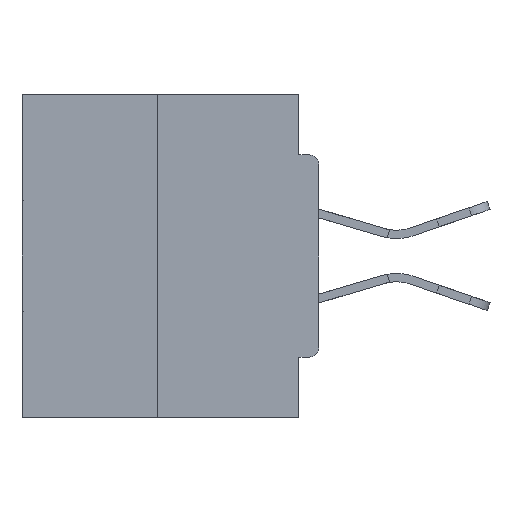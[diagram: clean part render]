
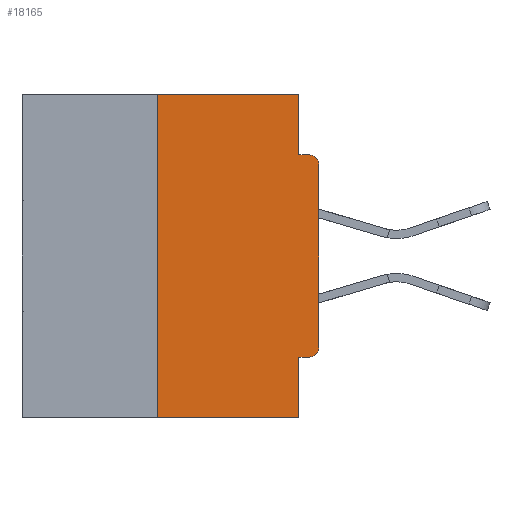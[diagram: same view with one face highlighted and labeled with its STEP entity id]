
A CAD part, left-side view. The second image highlights one B-rep face of the part: STEP entity #18165.
In plain terms, the highlighted planar face has unit normal (-1, 0, 0).
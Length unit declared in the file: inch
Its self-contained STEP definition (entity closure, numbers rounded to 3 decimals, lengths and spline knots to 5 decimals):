
#96 = VERTEX_POINT ( 'NONE', #27990 ) ;
#500 = DIRECTION ( 'NONE',  ( 0., -1., 0. ) ) ;
#645 = CIRCLE ( 'NONE', #2273, 0.015 ) ;
#762 = VECTOR ( 'NONE', #500, 39.37008 ) ;
#805 = VERTEX_POINT ( 'NONE', #32834 ) ;
#1297 = EDGE_CURVE ( 'NONE', #8215, #9489, #29503, .T. ) ;
#1760 = LINE ( 'NONE', #36639, #36650 ) ;
#1950 = EDGE_LOOP ( 'NONE', ( #38988, #21185, #4575, #33597, #34067, #13306, #17500, #25959, #10683, #33897 ) ) ;
#2273 = AXIS2_PLACEMENT_3D ( 'NONE', #25875, #7058, #6912 ) ;
#2349 = VERTEX_POINT ( 'NONE', #29491 ) ;
#2545 = VERTEX_POINT ( 'NONE', #11940 ) ;
#2670 = DIRECTION ( 'NONE',  ( 0., 0., -1. ) ) ;
#4311 = EDGE_CURVE ( 'NONE', #2545, #2349, #1760, .T. ) ;
#4575 = ORIENTED_EDGE ( 'NONE', *, *, #1297, .T. ) ;
#5375 = PLANE ( 'NONE',  #36277 ) ;
#5577 = AXIS2_PLACEMENT_3D ( 'NONE', #35127, #19532, #7070 ) ;
#5685 = LINE ( 'NONE', #37284, #11078 ) ;
#5915 = DIRECTION ( 'NONE',  ( 0., 0., 1. ) ) ;
#6201 = DIRECTION ( 'NONE',  ( 0., 1., 0. ) ) ;
#6490 = VECTOR ( 'NONE', #2670, 39.37008 ) ;
#6912 = DIRECTION ( 'NONE',  ( 0., 0., -1. ) ) ;
#7058 = DIRECTION ( 'NONE',  ( -1., 0., 0. ) ) ;
#7070 = DIRECTION ( 'NONE',  ( 0., 0., -1. ) ) ;
#8215 = VERTEX_POINT ( 'NONE', #9877 ) ;
#8361 = DIRECTION ( 'NONE',  ( 0., 0., -1. ) ) ;
#8403 = DIRECTION ( 'NONE',  ( 0., -1., 0. ) ) ;
#8501 = EDGE_CURVE ( 'NONE', #20234, #36156, #9989, .T. ) ;
#8911 = VERTEX_POINT ( 'NONE', #37414 ) ;
#9489 = VERTEX_POINT ( 'NONE', #32474 ) ;
#9556 = CARTESIAN_POINT ( 'NONE',  ( 0., 0.015, -0.0935 ) ) ;
#9877 = CARTESIAN_POINT ( 'NONE',  ( 0., 0.25, -0.5 ) ) ;
#9989 = CIRCLE ( 'NONE', #5577, 0.015 ) ;
#10274 = EDGE_CURVE ( 'NONE', #8911, #9489, #10868, .T. ) ;
#10683 = ORIENTED_EDGE ( 'NONE', *, *, #27005, .F. ) ;
#10868 = LINE ( 'NONE', #17713, #18225 ) ;
#11078 = VECTOR ( 'NONE', #5915, 39.37008 ) ;
#11924 = DIRECTION ( 'NONE',  ( 0., 0., -1. ) ) ;
#11940 = CARTESIAN_POINT ( 'NONE',  ( 0., 0.25, 0. ) ) ;
#13306 = ORIENTED_EDGE ( 'NONE', *, *, #8501, .T. ) ;
#13965 = EDGE_CURVE ( 'NONE', #36156, #96, #5685, .T. ) ;
#15790 = CARTESIAN_POINT ( 'NONE',  ( 0., 0., -0.4065 ) ) ;
#15932 = LINE ( 'NONE', #28334, #762 ) ;
#16157 = VECTOR ( 'NONE', #37316, 39.37008 ) ;
#16857 = CARTESIAN_POINT ( 'NONE',  ( 0., 0.25, 0. ) ) ;
#17297 = CARTESIAN_POINT ( 'NONE',  ( 0., 0., -0.3915 ) ) ;
#17500 = ORIENTED_EDGE ( 'NONE', *, *, #13965, .T. ) ;
#17713 = CARTESIAN_POINT ( 'NONE',  ( 0., 0.031, -0.5 ) ) ;
#17870 = DIRECTION ( 'NONE',  ( 1., 0., 0. ) ) ;
#18165 = ADVANCED_FACE ( 'NONE', ( #28165 ), #5375, .F. ) ;
#18225 = VECTOR ( 'NONE', #8361, 39.37008 ) ;
#19532 = DIRECTION ( 'NONE',  ( -1., 0., 0. ) ) ;
#20234 = VERTEX_POINT ( 'NONE', #31970 ) ;
#20324 = EDGE_CURVE ( 'NONE', #8215, #2545, #29466, .T. ) ;
#20418 = CARTESIAN_POINT ( 'NONE',  ( 0., 0.031, 0. ) ) ;
#21038 = VECTOR ( 'NONE', #35871, 39.37008 ) ;
#21185 = ORIENTED_EDGE ( 'NONE', *, *, #20324, .F. ) ;
#21501 = VECTOR ( 'NONE', #6201, 39.37008 ) ;
#24350 = CARTESIAN_POINT ( 'NONE',  ( 0., 0.46, 0. ) ) ;
#25875 = CARTESIAN_POINT ( 'NONE',  ( 0., 0.015, -0.1085 ) ) ;
#25959 = ORIENTED_EDGE ( 'NONE', *, *, #27768, .T. ) ;
#27005 = EDGE_CURVE ( 'NONE', #805, #29598, #15932, .T. ) ;
#27768 = EDGE_CURVE ( 'NONE', #96, #29598, #645, .T. ) ;
#27990 = CARTESIAN_POINT ( 'NONE',  ( 0., 0., -0.1085 ) ) ;
#28165 = FACE_OUTER_BOUND ( 'NONE', #1950, .T. ) ;
#28239 = EDGE_CURVE ( 'NONE', #2349, #805, #40003, .T. ) ;
#28334 = CARTESIAN_POINT ( 'NONE',  ( 0., 0., -0.0935 ) ) ;
#29466 = LINE ( 'NONE', #16857, #21038 ) ;
#29491 = CARTESIAN_POINT ( 'NONE',  ( 0., 0.031, 0. ) ) ;
#29503 = LINE ( 'NONE', #34169, #16157 ) ;
#29598 = VERTEX_POINT ( 'NONE', #9556 ) ;
#31970 = CARTESIAN_POINT ( 'NONE',  ( 0., 0.015, -0.4065 ) ) ;
#32474 = CARTESIAN_POINT ( 'NONE',  ( 0., 0.031, -0.5 ) ) ;
#32834 = CARTESIAN_POINT ( 'NONE',  ( 0., 0.031, -0.0935 ) ) ;
#33597 = ORIENTED_EDGE ( 'NONE', *, *, #10274, .F. ) ;
#33792 = EDGE_CURVE ( 'NONE', #20234, #8911, #34322, .T. ) ;
#33897 = ORIENTED_EDGE ( 'NONE', *, *, #28239, .F. ) ;
#34067 = ORIENTED_EDGE ( 'NONE', *, *, #33792, .F. ) ;
#34169 = CARTESIAN_POINT ( 'NONE',  ( 0., 0.46, -0.5 ) ) ;
#34322 = LINE ( 'NONE', #15790, #21501 ) ;
#35127 = CARTESIAN_POINT ( 'NONE',  ( 0., 0.015, -0.3915 ) ) ;
#35871 = DIRECTION ( 'NONE',  ( 0., 0., 1. ) ) ;
#36156 = VERTEX_POINT ( 'NONE', #17297 ) ;
#36277 = AXIS2_PLACEMENT_3D ( 'NONE', #24350, #17870, #11924 ) ;
#36639 = CARTESIAN_POINT ( 'NONE',  ( 0., 0.46, 0. ) ) ;
#36650 = VECTOR ( 'NONE', #8403, 39.37008 ) ;
#37284 = CARTESIAN_POINT ( 'NONE',  ( 0., 0., 0. ) ) ;
#37316 = DIRECTION ( 'NONE',  ( 0., -1., 0. ) ) ;
#37414 = CARTESIAN_POINT ( 'NONE',  ( 0., 0.031, -0.4065 ) ) ;
#38988 = ORIENTED_EDGE ( 'NONE', *, *, #4311, .F. ) ;
#40003 = LINE ( 'NONE', #20418, #6490 ) ;
